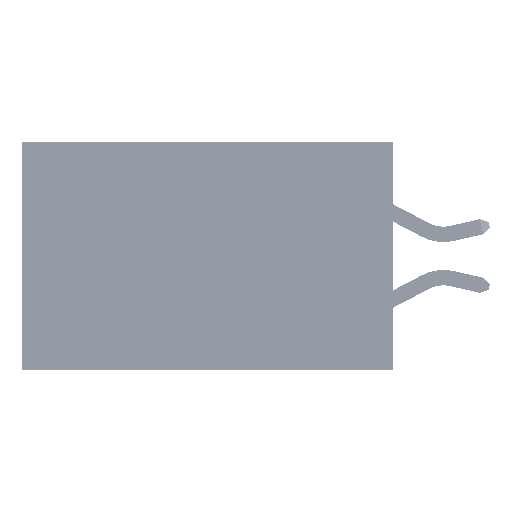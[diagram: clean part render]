
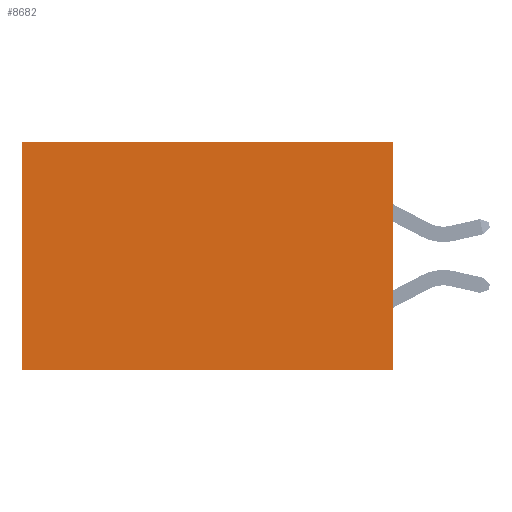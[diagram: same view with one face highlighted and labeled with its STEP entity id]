
A CAD part, left-side view. The second image highlights one B-rep face of the part: STEP entity #8682.
In plain terms, the highlighted planar face has unit normal (-1, 0, 0).
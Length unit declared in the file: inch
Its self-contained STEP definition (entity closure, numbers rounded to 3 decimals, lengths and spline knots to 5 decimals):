
#21 = VERTEX_POINT ( 'NONE', #10306 ) ;
#425 = VECTOR ( 'NONE', #31514, 39.37008 ) ;
#1052 = ORIENTED_EDGE ( 'NONE', *, *, #29607, .F. ) ;
#2886 = CARTESIAN_POINT ( 'NONE',  ( 0.2875, 0., 0. ) ) ;
#5313 = DIRECTION ( 'NONE',  ( 1., 0., 0. ) ) ;
#8620 = EDGE_CURVE ( 'NONE', #21, #33331, #44109, .T. ) ;
#8682 = ADVANCED_FACE ( 'NONE', ( #41941 ), #21276, .F. ) ;
#9978 = DIRECTION ( 'NONE',  ( 0., 1., 0. ) ) ;
#10306 = CARTESIAN_POINT ( 'NONE',  ( 0.2875, 0., -0.37 ) ) ;
#10391 = CARTESIAN_POINT ( 'NONE',  ( 0.2875, 0., 0. ) ) ;
#11399 = CARTESIAN_POINT ( 'NONE',  ( 0.2875, 0.6, -0.37 ) ) ;
#12220 = CARTESIAN_POINT ( 'NONE',  ( 0.2875, 0., 0. ) ) ;
#14031 = LINE ( 'NONE', #33227, #31227 ) ;
#14327 = EDGE_LOOP ( 'NONE', ( #41033, #36153, #1052, #22423 ) ) ;
#15523 = DIRECTION ( 'NONE',  ( 0., 0., -1. ) ) ;
#15527 = DIRECTION ( 'NONE',  ( 0., 0., -1. ) ) ;
#16523 = VERTEX_POINT ( 'NONE', #12220 ) ;
#19386 = VECTOR ( 'NONE', #41704, 39.37008 ) ;
#21276 = PLANE ( 'NONE',  #26045 ) ;
#22423 = ORIENTED_EDGE ( 'NONE', *, *, #26407, .T. ) ;
#26045 = AXIS2_PLACEMENT_3D ( 'NONE', #40043, #5313, #15527 ) ;
#26407 = EDGE_CURVE ( 'NONE', #16523, #28023, #34167, .T. ) ;
#28023 = VERTEX_POINT ( 'NONE', #28347 ) ;
#28347 = CARTESIAN_POINT ( 'NONE',  ( 0.2875, 0.6, 0. ) ) ;
#29607 = EDGE_CURVE ( 'NONE', #16523, #21, #32843, .T. ) ;
#31227 = VECTOR ( 'NONE', #15523, 39.37008 ) ;
#31514 = DIRECTION ( 'NONE',  ( 0., 1., 0. ) ) ;
#32843 = LINE ( 'NONE', #10391, #19386 ) ;
#33227 = CARTESIAN_POINT ( 'NONE',  ( 0.2875, 0.6, 0. ) ) ;
#33331 = VERTEX_POINT ( 'NONE', #11399 ) ;
#34167 = LINE ( 'NONE', #2886, #44442 ) ;
#35260 = CARTESIAN_POINT ( 'NONE',  ( 0.2875, 0., -0.37 ) ) ;
#36153 = ORIENTED_EDGE ( 'NONE', *, *, #8620, .F. ) ;
#38656 = EDGE_CURVE ( 'NONE', #28023, #33331, #14031, .T. ) ;
#40043 = CARTESIAN_POINT ( 'NONE',  ( 0.2875, 0., 0. ) ) ;
#41033 = ORIENTED_EDGE ( 'NONE', *, *, #38656, .T. ) ;
#41704 = DIRECTION ( 'NONE',  ( 0., 0., -1. ) ) ;
#41941 = FACE_OUTER_BOUND ( 'NONE', #14327, .T. ) ;
#44109 = LINE ( 'NONE', #35260, #425 ) ;
#44442 = VECTOR ( 'NONE', #9978, 39.37008 ) ;
